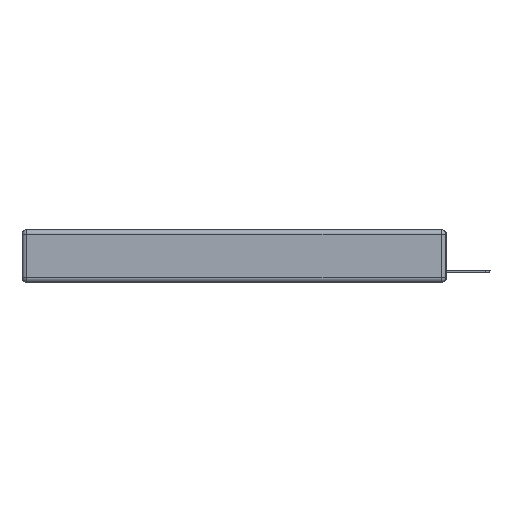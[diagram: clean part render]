
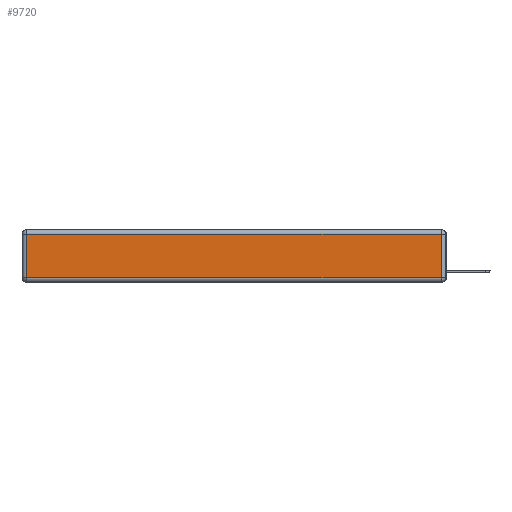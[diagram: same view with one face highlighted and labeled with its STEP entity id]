
A CAD part, left-side view. The second image highlights one B-rep face of the part: STEP entity #9720.
In plain terms, the highlighted planar face has unit normal (-1, 0, 0).
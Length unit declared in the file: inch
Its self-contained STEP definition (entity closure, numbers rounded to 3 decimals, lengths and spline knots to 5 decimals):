
#410 = DIRECTION ( 'NONE',  ( 0., 0., -1. ) ) ;
#889 = CARTESIAN_POINT ( 'NONE',  ( 0., 2.72, -0.343 ) ) ;
#1626 = CARTESIAN_POINT ( 'NONE',  ( 0., 0., -0.343 ) ) ;
#1840 = ORIENTED_EDGE ( 'NONE', *, *, #13687, .T. ) ;
#1988 = ORIENTED_EDGE ( 'NONE', *, *, #21586, .T. ) ;
#2670 = CARTESIAN_POINT ( 'NONE',  ( 0., 2.72, -0.313 ) ) ;
#2951 = VERTEX_POINT ( 'NONE', #9837 ) ;
#3284 = EDGE_CURVE ( 'NONE', #2951, #14205, #7137, .T. ) ;
#3658 = ORIENTED_EDGE ( 'NONE', *, *, #3284, .T. ) ;
#7137 = LINE ( 'NONE', #7252, #18698 ) ;
#7252 = CARTESIAN_POINT ( 'NONE',  ( 0., 0.03, -0.343 ) ) ;
#7355 = DIRECTION ( 'NONE',  ( 0., 0., 1. ) ) ;
#7383 = CARTESIAN_POINT ( 'NONE',  ( 0., 0., -0.313 ) ) ;
#9014 = ORIENTED_EDGE ( 'NONE', *, *, #11959, .T. ) ;
#9211 = VERTEX_POINT ( 'NONE', #2670 ) ;
#9664 = VECTOR ( 'NONE', #410, 39.37008 ) ;
#9720 = ADVANCED_FACE ( 'NONE', ( #12956 ), #11000, .T. ) ;
#9837 = CARTESIAN_POINT ( 'NONE',  ( 0., 0.03, -0.313 ) ) ;
#10032 = VECTOR ( 'NONE', #13599, 39.37008 ) ;
#10145 = LINE ( 'NONE', #889, #9664 ) ;
#10362 = CARTESIAN_POINT ( 'NONE',  ( 0., 2.72, -0.03 ) ) ;
#11000 = PLANE ( 'NONE',  #14635 ) ;
#11959 = EDGE_CURVE ( 'NONE', #14205, #19245, #18935, .T. ) ;
#12956 = FACE_OUTER_BOUND ( 'NONE', #18367, .T. ) ;
#13599 = DIRECTION ( 'NONE',  ( 0., 1., 0. ) ) ;
#13687 = EDGE_CURVE ( 'NONE', #19245, #9211, #10145, .T. ) ;
#14205 = VERTEX_POINT ( 'NONE', #19934 ) ;
#14635 = AXIS2_PLACEMENT_3D ( 'NONE', #1626, #21844, #7355 ) ;
#15543 = CARTESIAN_POINT ( 'NONE',  ( 0., 2.75, -0.03 ) ) ;
#16748 = LINE ( 'NONE', #7383, #17370 ) ;
#17370 = VECTOR ( 'NONE', #20636, 39.37008 ) ;
#18367 = EDGE_LOOP ( 'NONE', ( #1988, #3658, #9014, #1840 ) ) ;
#18698 = VECTOR ( 'NONE', #20046, 39.37008 ) ;
#18935 = LINE ( 'NONE', #15543, #10032 ) ;
#19245 = VERTEX_POINT ( 'NONE', #10362 ) ;
#19934 = CARTESIAN_POINT ( 'NONE',  ( 0., 0.03, -0.03 ) ) ;
#20046 = DIRECTION ( 'NONE',  ( 0., 0., 1. ) ) ;
#20636 = DIRECTION ( 'NONE',  ( 0., -1., 0. ) ) ;
#21586 = EDGE_CURVE ( 'NONE', #9211, #2951, #16748, .T. ) ;
#21844 = DIRECTION ( 'NONE',  ( -1., 0., 0. ) ) ;
